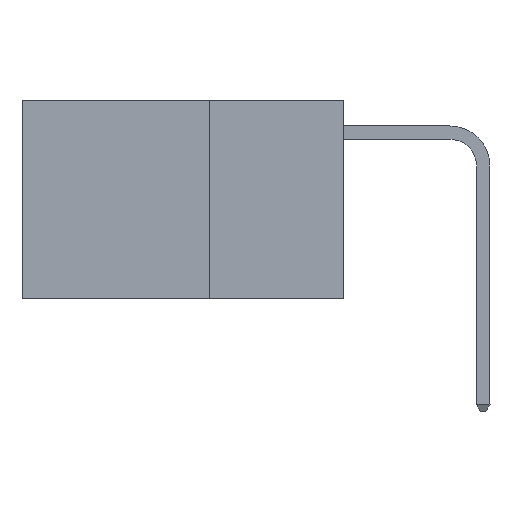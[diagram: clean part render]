
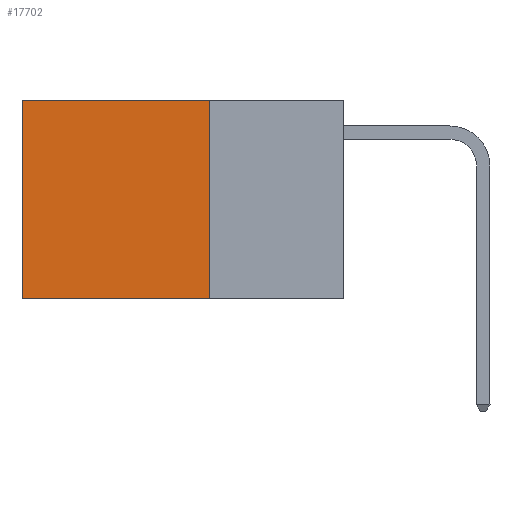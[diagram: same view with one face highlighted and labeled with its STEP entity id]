
A CAD part, left-side view. The second image highlights one B-rep face of the part: STEP entity #17702.
In plain terms, the highlighted planar face has unit normal (-1, 0, 0).
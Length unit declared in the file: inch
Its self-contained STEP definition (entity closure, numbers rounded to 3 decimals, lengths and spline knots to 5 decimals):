
#6 = LINE ( 'NONE', #18172, #11062 ) ;
#1185 = CARTESIAN_POINT ( 'NONE',  ( 0.2625, 0.25, 0. ) ) ;
#1334 = DIRECTION ( 'NONE',  ( 0., 0., -1. ) ) ;
#1540 = EDGE_CURVE ( 'NONE', #16931, #12173, #10375, .T. ) ;
#1781 = FACE_OUTER_BOUND ( 'NONE', #2345, .T. ) ;
#2034 = LINE ( 'NONE', #6888, #15712 ) ;
#2037 = CARTESIAN_POINT ( 'NONE',  ( 0.2625, 0.25, -0.37 ) ) ;
#2184 = VERTEX_POINT ( 'NONE', #8553 ) ;
#2341 = ORIENTED_EDGE ( 'NONE', *, *, #16986, .F. ) ;
#2345 = EDGE_LOOP ( 'NONE', ( #5646, #2341, #9037, #7863 ) ) ;
#2459 = CARTESIAN_POINT ( 'NONE',  ( 0.2625, 0.25, 0. ) ) ;
#2650 = DIRECTION ( 'NONE',  ( 0., 0., -1. ) ) ;
#3850 = EDGE_CURVE ( 'NONE', #12173, #2184, #12407, .T. ) ;
#3911 = CARTESIAN_POINT ( 'NONE',  ( 0.2625, 0.25, 0. ) ) ;
#3947 = DIRECTION ( 'NONE',  ( 0., 0., -1. ) ) ;
#4521 = AXIS2_PLACEMENT_3D ( 'NONE', #1185, #11200, #2650 ) ;
#5646 = ORIENTED_EDGE ( 'NONE', *, *, #3850, .T. ) ;
#6610 = VECTOR ( 'NONE', #16556, 39.37008 ) ;
#6888 = CARTESIAN_POINT ( 'NONE',  ( 0.2625, 0.25, -0.37 ) ) ;
#7863 = ORIENTED_EDGE ( 'NONE', *, *, #1540, .T. ) ;
#8339 = PLANE ( 'NONE',  #4521 ) ;
#8553 = CARTESIAN_POINT ( 'NONE',  ( 0.2625, 0.6, -0.37 ) ) ;
#9037 = ORIENTED_EDGE ( 'NONE', *, *, #15268, .F. ) ;
#10375 = LINE ( 'NONE', #2459, #6610 ) ;
#11062 = VECTOR ( 'NONE', #1334, 39.37008 ) ;
#11200 = DIRECTION ( 'NONE',  ( 1., 0., 0. ) ) ;
#12173 = VERTEX_POINT ( 'NONE', #16107 ) ;
#12407 = LINE ( 'NONE', #13771, #16487 ) ;
#13659 = VERTEX_POINT ( 'NONE', #2037 ) ;
#13771 = CARTESIAN_POINT ( 'NONE',  ( 0.2625, 0.6, 0. ) ) ;
#15268 = EDGE_CURVE ( 'NONE', #16931, #13659, #6, .T. ) ;
#15712 = VECTOR ( 'NONE', #16642, 39.37008 ) ;
#16107 = CARTESIAN_POINT ( 'NONE',  ( 0.2625, 0.6, 0. ) ) ;
#16487 = VECTOR ( 'NONE', #3947, 39.37008 ) ;
#16556 = DIRECTION ( 'NONE',  ( 0., 1., 0. ) ) ;
#16642 = DIRECTION ( 'NONE',  ( 0., 1., 0. ) ) ;
#16931 = VERTEX_POINT ( 'NONE', #3911 ) ;
#16986 = EDGE_CURVE ( 'NONE', #13659, #2184, #2034, .T. ) ;
#17702 = ADVANCED_FACE ( 'NONE', ( #1781 ), #8339, .F. ) ;
#18172 = CARTESIAN_POINT ( 'NONE',  ( 0.2625, 0.25, 0. ) ) ;
